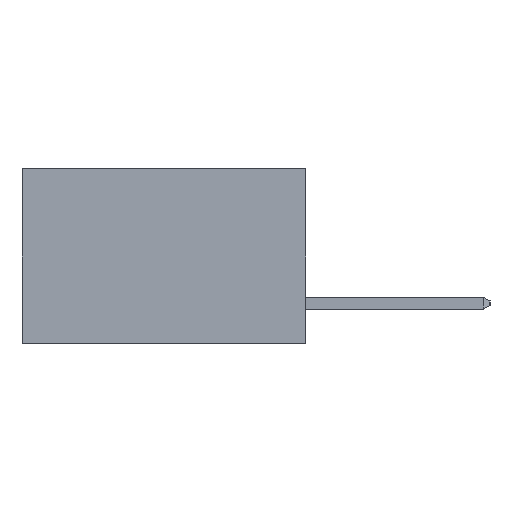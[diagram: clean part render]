
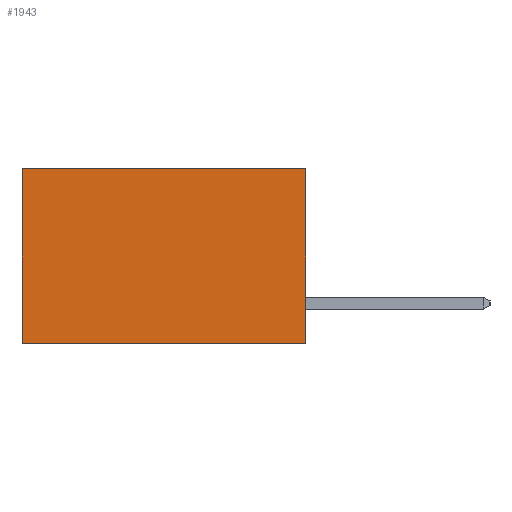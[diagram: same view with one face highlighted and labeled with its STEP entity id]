
A CAD part, left-side view. The second image highlights one B-rep face of the part: STEP entity #1943.
In plain terms, the highlighted planar face has unit normal (-1, 0, 0).
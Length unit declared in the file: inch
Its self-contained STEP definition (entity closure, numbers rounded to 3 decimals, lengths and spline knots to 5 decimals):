
#253 = CARTESIAN_POINT ( 'NONE',  ( 0.2615, 0., -0.37 ) ) ;
#347 = ORIENTED_EDGE ( 'NONE', *, *, #677, .F. ) ;
#677 = EDGE_CURVE ( 'NONE', #1951, #4015, #6029, .T. ) ;
#716 = VECTOR ( 'NONE', #9691, 39.37008 ) ;
#1794 = CARTESIAN_POINT ( 'NONE',  ( 0.2615, 0., -0.37 ) ) ;
#1943 = ADVANCED_FACE ( 'NONE', ( #13040 ), #9767, .F. ) ;
#1951 = VERTEX_POINT ( 'NONE', #7184 ) ;
#2079 = VECTOR ( 'NONE', #2414, 39.37008 ) ;
#2111 = ORIENTED_EDGE ( 'NONE', *, *, #12518, .T. ) ;
#2177 = EDGE_CURVE ( 'NONE', #4015, #4056, #7228, .T. ) ;
#2414 = DIRECTION ( 'NONE',  ( 0., 0., -1. ) ) ;
#2786 = CARTESIAN_POINT ( 'NONE',  ( 0.2615, 0., 0. ) ) ;
#3111 = ORIENTED_EDGE ( 'NONE', *, *, #10972, .T. ) ;
#3227 = CARTESIAN_POINT ( 'NONE',  ( 0.2615, 0., -0.37 ) ) ;
#3892 = LINE ( 'NONE', #2786, #716 ) ;
#4015 = VERTEX_POINT ( 'NONE', #6608 ) ;
#4056 = VERTEX_POINT ( 'NONE', #4336 ) ;
#4336 = CARTESIAN_POINT ( 'NONE',  ( 0.2615, 0.6, -0.37 ) ) ;
#4829 = DIRECTION ( 'NONE',  ( 0., 1., 0. ) ) ;
#5603 = VERTEX_POINT ( 'NONE', #12956 ) ;
#5918 = CARTESIAN_POINT ( 'NONE',  ( 0.2615, 0.6, -0.37 ) ) ;
#6029 = LINE ( 'NONE', #1794, #11690 ) ;
#6608 = CARTESIAN_POINT ( 'NONE',  ( 0.2615, 0., -0.37 ) ) ;
#7184 = CARTESIAN_POINT ( 'NONE',  ( 0.2615, 0., 0. ) ) ;
#7228 = LINE ( 'NONE', #3227, #12848 ) ;
#7868 = AXIS2_PLACEMENT_3D ( 'NONE', #253, #12904, #14772 ) ;
#8247 = LINE ( 'NONE', #5918, #2079 ) ;
#9485 = EDGE_LOOP ( 'NONE', ( #3111, #12027, #347, #2111 ) ) ;
#9691 = DIRECTION ( 'NONE',  ( 0., 1., 0. ) ) ;
#9767 = PLANE ( 'NONE',  #7868 ) ;
#10972 = EDGE_CURVE ( 'NONE', #5603, #4056, #8247, .T. ) ;
#11338 = DIRECTION ( 'NONE',  ( 0., 0., -1. ) ) ;
#11690 = VECTOR ( 'NONE', #11338, 39.37008 ) ;
#12027 = ORIENTED_EDGE ( 'NONE', *, *, #2177, .F. ) ;
#12518 = EDGE_CURVE ( 'NONE', #1951, #5603, #3892, .T. ) ;
#12848 = VECTOR ( 'NONE', #4829, 39.37008 ) ;
#12904 = DIRECTION ( 'NONE',  ( 1., 0., 0. ) ) ;
#12956 = CARTESIAN_POINT ( 'NONE',  ( 0.2615, 0.6, 0. ) ) ;
#13040 = FACE_OUTER_BOUND ( 'NONE', #9485, .T. ) ;
#14772 = DIRECTION ( 'NONE',  ( 0., 0., -1. ) ) ;
